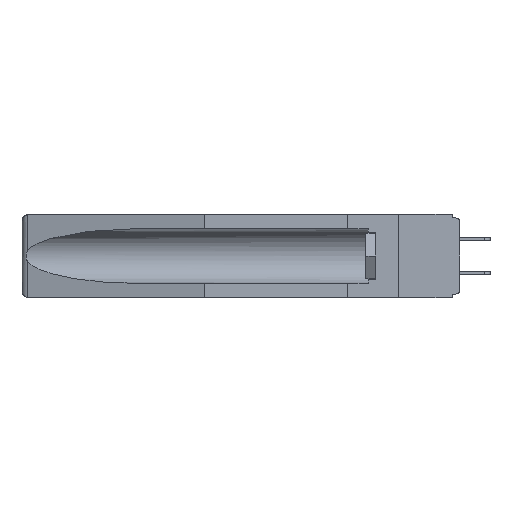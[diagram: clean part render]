
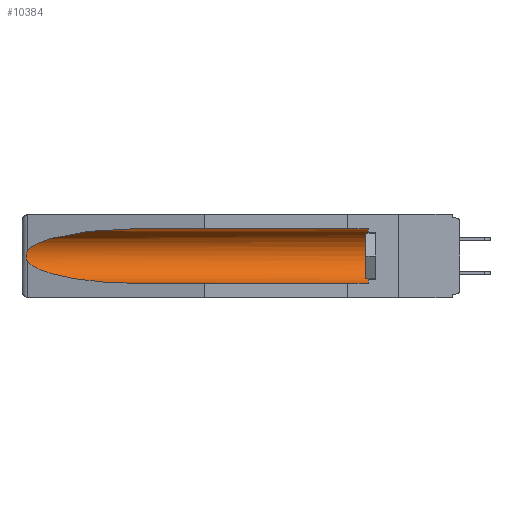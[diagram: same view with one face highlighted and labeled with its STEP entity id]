
A CAD part, left-side view. The second image highlights one B-rep face of the part: STEP entity #10384.
In plain terms, the highlighted cylindrical face has radius 2.857 mm (diameter 5.715 mm), a partial arc.
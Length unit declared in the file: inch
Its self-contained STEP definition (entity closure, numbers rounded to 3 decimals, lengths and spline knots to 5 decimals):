
#213 = ORIENTED_EDGE ( 'NONE', *, *, #6664, .T. ) ;
#804 = CARTESIAN_POINT ( 'NONE',  ( 0.26537, 1.52718, -0.14972 ) ) ;
#815 = DIRECTION ( 'NONE',  ( 0., 0., 1. ) ) ;
#972 = CIRCLE ( 'NONE', #12532, 0.1125 ) ;
#1210 = CARTESIAN_POINT ( 'NONE',  ( 0.25451, 1.48313, -0.24835 ) ) ;
#1387 = FACE_OUTER_BOUND ( 'NONE', #9547, .T. ) ;
#1678 = CARTESIAN_POINT ( 'NONE',  ( 0.155, 1.07973, -0.059 ) ) ;
#1717 = CARTESIAN_POINT ( 'NONE',  ( 0.155, 0.126, -0.1715 ) ) ;
#2280 = EDGE_CURVE ( 'NONE', #16817, #6842, #13527, .T. ) ;
#3518 = ORIENTED_EDGE ( 'NONE', *, *, #11398, .T. ) ;
#3646 = VECTOR ( 'NONE', #8604, 39.37008 ) ;
#3651 = CARTESIAN_POINT ( 'NONE',  ( 0.26655, 1.53094, -0.18657 ) ) ;
#3717 = CARTESIAN_POINT ( 'NONE',  ( 0.2675, 1.53308, -0.16763 ) ) ;
#3855 = LINE ( 'NONE', #15411, #3646 ) ;
#3898 = CARTESIAN_POINT ( 'NONE',  ( 0.155, -0.30754, -0.059 ) ) ;
#3950 = DIRECTION ( 'NONE',  ( 0., 1., 0. ) ) ;
#4155 = VECTOR ( 'NONE', #3950, 39.37008 ) ;
#4585 = ORIENTED_EDGE ( 'NONE', *, *, #2280, .T. ) ;
#4618 = CARTESIAN_POINT ( 'NONE',  ( 0.21114, 1.30732, -0.059 ) ) ;
#4661 = VERTEX_POINT ( 'NONE', #14257 ) ;
#4954 = CARTESIAN_POINT ( 'NONE',  ( 0.155, 1.07973, -0.284 ) ) ;
#5247 = CARTESIAN_POINT ( 'NONE',  ( 0.21114, 1.30732, -0.284 ) ) ;
#5435 = CARTESIAN_POINT ( 'NONE',  ( 0.155, 1.07973, -0.284 ) ) ;
#6196 = DIRECTION ( 'NONE',  ( 0., 1., 0. ) ) ;
#6664 = EDGE_CURVE ( 'NONE', #16538, #16817, #972, .T. ) ;
#6738 = EDGE_CURVE ( 'NONE', #6842, #8235, #15123, .T. ) ;
#6741 =( BOUNDED_CURVE ( )  B_SPLINE_CURVE ( 3, ( #13619, #1210, #5247, #5435 ),
 .UNSPECIFIED., .F., .F. ) 
 B_SPLINE_CURVE_WITH_KNOTS ( ( 4, 4 ),
 ( 0.1948, 1.5708 ),
 .UNSPECIFIED. ) 
 CURVE ( )  GEOMETRIC_REPRESENTATION_ITEM ( )  RATIONAL_B_SPLINE_CURVE ( ( 1., 0.848, 0.848, 1. ) ) 
 REPRESENTATION_ITEM ( '' )  );
#6842 = VERTEX_POINT ( 'NONE', #1678 ) ;
#7456 = CARTESIAN_POINT ( 'NONE',  ( 0.155, 0.126, -0.059 ) ) ;
#7528 = B_SPLINE_CURVE_WITH_KNOTS ( 'NONE', 3,
 ( #804, #10529, #17617, #9252, #3717, #8035, #13451, #3651, #14894, #10878 ),
 .UNSPECIFIED., .F., .F.,
 ( 4, 2, 2, 2, 4 ),
 ( 0., 0.00029, 0.00058, 0.00087, 0.00117 ),
 .UNSPECIFIED. ) ;
#7547 = ORIENTED_EDGE ( 'NONE', *, *, #9417, .T. ) ;
#8035 = CARTESIAN_POINT ( 'NONE',  ( 0.2675, 1.53308, -0.17534 ) ) ;
#8235 = VERTEX_POINT ( 'NONE', #15952 ) ;
#8604 = DIRECTION ( 'NONE',  ( 0., 1., 0. ) ) ;
#8845 = CARTESIAN_POINT ( 'NONE',  ( 0.26537, 1.52718, -0.14972 ) ) ;
#8904 = VERTEX_POINT ( 'NONE', #4954 ) ;
#9196 = ORIENTED_EDGE ( 'NONE', *, *, #6738, .T. ) ;
#9252 = CARTESIAN_POINT ( 'NONE',  ( 0.2673, 1.5327, -0.16383 ) ) ;
#9417 = EDGE_CURVE ( 'NONE', #8235, #4661, #7528, .T. ) ;
#9547 = EDGE_LOOP ( 'NONE', ( #9196, #7547, #3518, #15868, #213, #4585 ) ) ;
#10384 = ADVANCED_FACE ( 'NONE', ( #1387 ), #15309, .F. ) ;
#10529 = CARTESIAN_POINT ( 'NONE',  ( 0.26597, 1.52961, -0.15275 ) ) ;
#10878 = CARTESIAN_POINT ( 'NONE',  ( 0.26537, 1.52718, -0.19328 ) ) ;
#11398 = EDGE_CURVE ( 'NONE', #4661, #8904, #6741, .T. ) ;
#11585 = CARTESIAN_POINT ( 'NONE',  ( 0.155, 1.07973, -0.059 ) ) ;
#11703 = CARTESIAN_POINT ( 'NONE',  ( 0.155, -0.30754, -0.1715 ) ) ;
#12532 = AXIS2_PLACEMENT_3D ( 'NONE', #1717, #15662, #15833 ) ;
#12927 = CARTESIAN_POINT ( 'NONE',  ( 0.25451, 1.48313, -0.09465 ) ) ;
#13194 = EDGE_CURVE ( 'NONE', #16538, #8904, #3855, .T. ) ;
#13451 = CARTESIAN_POINT ( 'NONE',  ( 0.2673, 1.53269, -0.17917 ) ) ;
#13527 = LINE ( 'NONE', #3898, #4155 ) ;
#13528 = AXIS2_PLACEMENT_3D ( 'NONE', #11703, #6196, #815 ) ;
#13619 = CARTESIAN_POINT ( 'NONE',  ( 0.26537, 1.52718, -0.19328 ) ) ;
#14257 = CARTESIAN_POINT ( 'NONE',  ( 0.26537, 1.52718, -0.19328 ) ) ;
#14894 = CARTESIAN_POINT ( 'NONE',  ( 0.26597, 1.5296, -0.19026 ) ) ;
#15123 =( BOUNDED_CURVE ( )  B_SPLINE_CURVE ( 3, ( #11585, #4618, #12927, #8845 ),
 .UNSPECIFIED., .F., .F. ) 
 B_SPLINE_CURVE_WITH_KNOTS ( ( 4, 4 ),
 ( 4.71239, 6.08839 ),
 .UNSPECIFIED. ) 
 CURVE ( )  GEOMETRIC_REPRESENTATION_ITEM ( )  RATIONAL_B_SPLINE_CURVE ( ( 1., 0.848, 0.848, 1. ) ) 
 REPRESENTATION_ITEM ( '' )  );
#15309 = CYLINDRICAL_SURFACE ( 'NONE', #13528, 0.1125 ) ;
#15411 = CARTESIAN_POINT ( 'NONE',  ( 0.155, -0.30754, -0.284 ) ) ;
#15662 = DIRECTION ( 'NONE',  ( 0., -1., 0. ) ) ;
#15833 = DIRECTION ( 'NONE',  ( 0., 0., 1. ) ) ;
#15868 = ORIENTED_EDGE ( 'NONE', *, *, #13194, .F. ) ;
#15952 = CARTESIAN_POINT ( 'NONE',  ( 0.26537, 1.52718, -0.14972 ) ) ;
#16538 = VERTEX_POINT ( 'NONE', #16734 ) ;
#16734 = CARTESIAN_POINT ( 'NONE',  ( 0.155, 0.126, -0.284 ) ) ;
#16817 = VERTEX_POINT ( 'NONE', #7456 ) ;
#17617 = CARTESIAN_POINT ( 'NONE',  ( 0.26654, 1.53092, -0.15636 ) ) ;
